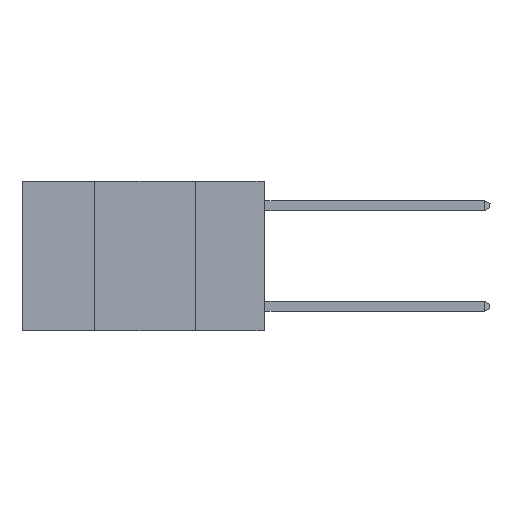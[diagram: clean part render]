
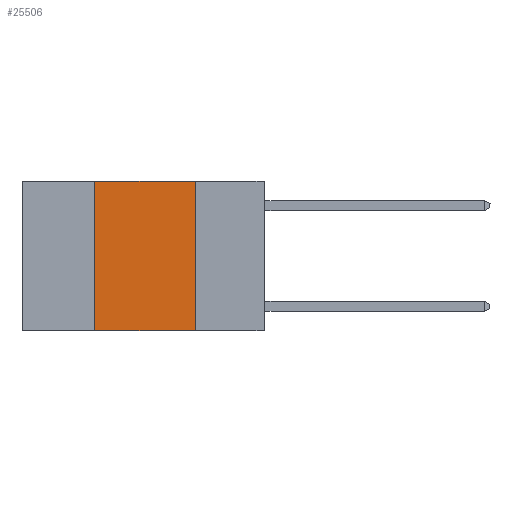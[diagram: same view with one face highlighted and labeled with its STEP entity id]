
A CAD part, left-side view. The second image highlights one B-rep face of the part: STEP entity #25506.
In plain terms, the highlighted planar face has unit normal (-1, 0, 0).
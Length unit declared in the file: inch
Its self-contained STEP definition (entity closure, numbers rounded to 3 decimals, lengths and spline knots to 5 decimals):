
#103 = PLANE ( 'NONE',  #1701 ) ;
#517 = DIRECTION ( 'NONE',  ( 0., 0., -1. ) ) ;
#638 = EDGE_CURVE ( 'NONE', #29685, #6369, #18861, .T. ) ;
#1701 = AXIS2_PLACEMENT_3D ( 'NONE', #17448, #25479, #26345 ) ;
#2187 = CARTESIAN_POINT ( 'NONE',  ( 0., 0.42, -0.37 ) ) ;
#2917 = CARTESIAN_POINT ( 'NONE',  ( 0., 0.42, 0. ) ) ;
#3622 = ORIENTED_EDGE ( 'NONE', *, *, #638, .F. ) ;
#3702 = VECTOR ( 'NONE', #517, 39.37008 ) ;
#4511 = EDGE_LOOP ( 'NONE', ( #8359, #3622, #9964, #13353 ) ) ;
#6369 = VERTEX_POINT ( 'NONE', #10004 ) ;
#7056 = VECTOR ( 'NONE', #12241, 39.37008 ) ;
#7091 = CARTESIAN_POINT ( 'NONE',  ( 0., 0.17, 0. ) ) ;
#7176 = LINE ( 'NONE', #11761, #16394 ) ;
#7541 = VERTEX_POINT ( 'NONE', #22885 ) ;
#8359 = ORIENTED_EDGE ( 'NONE', *, *, #9551, .F. ) ;
#9551 = EDGE_CURVE ( 'NONE', #6369, #7541, #18708, .T. ) ;
#9964 = ORIENTED_EDGE ( 'NONE', *, *, #23486, .F. ) ;
#10004 = CARTESIAN_POINT ( 'NONE',  ( 0., 0.17, 0. ) ) ;
#11761 = CARTESIAN_POINT ( 'NONE',  ( 0., 0.6, -0.37 ) ) ;
#12241 = DIRECTION ( 'NONE',  ( 0., 0., 1. ) ) ;
#13353 = ORIENTED_EDGE ( 'NONE', *, *, #26401, .T. ) ;
#13817 = DIRECTION ( 'NONE',  ( 0., -1., 0. ) ) ;
#16159 = FACE_OUTER_BOUND ( 'NONE', #4511, .T. ) ;
#16394 = VECTOR ( 'NONE', #25517, 39.37008 ) ;
#16598 = VERTEX_POINT ( 'NONE', #2187 ) ;
#17448 = CARTESIAN_POINT ( 'NONE',  ( 0., 0.6, 0. ) ) ;
#18708 = LINE ( 'NONE', #7091, #3702 ) ;
#18861 = LINE ( 'NONE', #25438, #19163 ) ;
#19163 = VECTOR ( 'NONE', #13817, 39.37008 ) ;
#22885 = CARTESIAN_POINT ( 'NONE',  ( 0., 0.17, -0.37 ) ) ;
#23486 = EDGE_CURVE ( 'NONE', #16598, #29685, #23854, .T. ) ;
#23854 = LINE ( 'NONE', #2917, #7056 ) ;
#25438 = CARTESIAN_POINT ( 'NONE',  ( 0., 0.6, 0. ) ) ;
#25479 = DIRECTION ( 'NONE',  ( 1., 0., 0. ) ) ;
#25506 = ADVANCED_FACE ( 'NONE', ( #16159 ), #103, .F. ) ;
#25517 = DIRECTION ( 'NONE',  ( 0., -1., 0. ) ) ;
#26345 = DIRECTION ( 'NONE',  ( 0., 0., -1. ) ) ;
#26401 = EDGE_CURVE ( 'NONE', #16598, #7541, #7176, .T. ) ;
#27710 = CARTESIAN_POINT ( 'NONE',  ( 0., 0.42, 0. ) ) ;
#29685 = VERTEX_POINT ( 'NONE', #27710 ) ;
